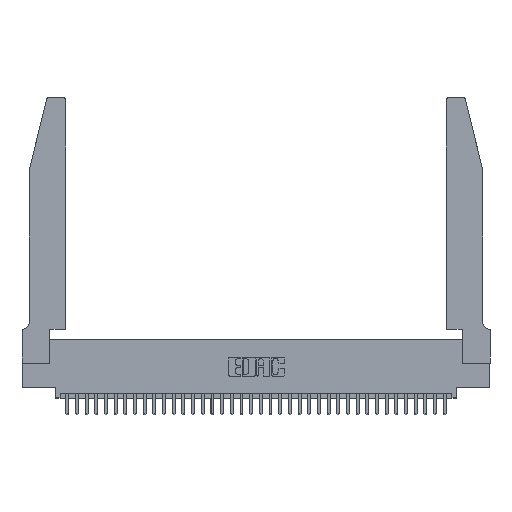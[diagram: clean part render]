
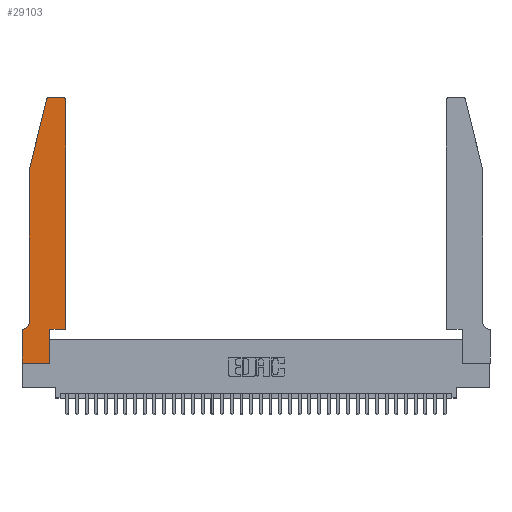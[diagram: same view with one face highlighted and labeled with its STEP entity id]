
A CAD part, top view. The second image highlights one B-rep face of the part: STEP entity #29103.
In plain terms, the highlighted planar face has unit normal (0, 0, 1).
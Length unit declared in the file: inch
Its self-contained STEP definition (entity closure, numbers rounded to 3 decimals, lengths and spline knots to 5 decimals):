
#94 = DIRECTION ( 'NONE',  ( -1., 0., 0. ) ) ;
#279 = CIRCLE ( 'NONE', #34975, 0.03 ) ;
#625 = FACE_OUTER_BOUND ( 'NONE', #15405, .T. ) ;
#995 = CARTESIAN_POINT ( 'NONE',  ( 0.0755, 2., 0.37 ) ) ;
#1442 = VECTOR ( 'NONE', #24357, 39.37008 ) ;
#2743 = DIRECTION ( 'NONE',  ( 0., 0., 1. ) ) ;
#3108 = CARTESIAN_POINT ( 'NONE',  ( 0.0755, 0.42, 0.37 ) ) ;
#3677 = LINE ( 'NONE', #20030, #7266 ) ;
#3759 = LINE ( 'NONE', #19079, #30808 ) ;
#3916 = LINE ( 'NONE', #7565, #27841 ) ;
#4178 = AXIS2_PLACEMENT_3D ( 'NONE', #19629, #25733, #22561 ) ;
#4283 = DIRECTION ( 'NONE',  ( 1., 0., 0. ) ) ;
#4795 = AXIS2_PLACEMENT_3D ( 'NONE', #17708, #6843, #6454 ) ;
#5957 = VECTOR ( 'NONE', #19794, 39.37008 ) ;
#6454 = DIRECTION ( 'NONE',  ( -1., 0., 0. ) ) ;
#6843 = DIRECTION ( 'NONE',  ( 0., 0., -1. ) ) ;
#7266 = VECTOR ( 'NONE', #11717, 39.37008 ) ;
#7565 = CARTESIAN_POINT ( 'NONE',  ( 0.4505, 0.35, 0.37 ) ) ;
#8391 = VERTEX_POINT ( 'NONE', #36003 ) ;
#9439 = EDGE_CURVE ( 'NONE', #10464, #17685, #34648, .T. ) ;
#9885 = DIRECTION ( 'NONE',  ( 0., 1., 0. ) ) ;
#10156 = ORIENTED_EDGE ( 'NONE', *, *, #19730, .T. ) ;
#10464 = VERTEX_POINT ( 'NONE', #36129 ) ;
#10573 = ORIENTED_EDGE ( 'NONE', *, *, #26274, .T. ) ;
#10985 = ORIENTED_EDGE ( 'NONE', *, *, #24171, .T. ) ;
#11085 = LINE ( 'NONE', #34331, #11903 ) ;
#11710 = ORIENTED_EDGE ( 'NONE', *, *, #30419, .T. ) ;
#11717 = DIRECTION ( 'NONE',  ( -1., 0., 0. ) ) ;
#11903 = VECTOR ( 'NONE', #17956, 39.37008 ) ;
#12091 = ORIENTED_EDGE ( 'NONE', *, *, #30946, .T. ) ;
#12439 = CARTESIAN_POINT ( 'NONE',  ( 0.4505, 0.35, 0.37 ) ) ;
#12511 = EDGE_CURVE ( 'NONE', #17685, #28322, #3916, .T. ) ;
#12722 = VERTEX_POINT ( 'NONE', #17600 ) ;
#12914 = LINE ( 'NONE', #30201, #31939 ) ;
#13151 = DIRECTION ( 'NONE',  ( 0., -1., 0. ) ) ;
#13572 = CARTESIAN_POINT ( 'NONE',  ( 0.25487, 2.72718, 0.37 ) ) ;
#13849 = DIRECTION ( 'NONE',  ( 1., 0., 0. ) ) ;
#13865 = CIRCLE ( 'NONE', #4795, 0.07 ) ;
#13953 = CARTESIAN_POINT ( 'NONE',  ( 0.284, 2.72, 0.37 ) ) ;
#14131 = VECTOR ( 'NONE', #94, 39.37008 ) ;
#14775 = EDGE_CURVE ( 'NONE', #35004, #17562, #3759, .T. ) ;
#15405 = EDGE_LOOP ( 'NONE', ( #11710, #12091, #22110, #30560, #10985, #10573, #32039, #10156, #29866, #31590, #23217, #34925 ) ) ;
#16206 = DIRECTION ( 'NONE',  ( -0.239, -0.971, 0. ) ) ;
#16333 = CARTESIAN_POINT ( 'NONE',  ( 0.0055, 0.35, 0.37 ) ) ;
#16591 = CARTESIAN_POINT ( 'NONE',  ( 0., 0.35, 0.37 ) ) ;
#16784 = VERTEX_POINT ( 'NONE', #16333 ) ;
#17246 = CARTESIAN_POINT ( 'NONE',  ( 0.0755, 0.35, 0.37 ) ) ;
#17562 = VERTEX_POINT ( 'NONE', #995 ) ;
#17600 = CARTESIAN_POINT ( 'NONE',  ( 0.4205, 2.75, 0.37 ) ) ;
#17685 = VERTEX_POINT ( 'NONE', #12439 ) ;
#17708 = CARTESIAN_POINT ( 'NONE',  ( 0.0055, 0.42, 0.37 ) ) ;
#17956 = DIRECTION ( 'NONE',  ( 0., 1., 0. ) ) ;
#18229 = EDGE_CURVE ( 'NONE', #28322, #12722, #279, .T. ) ;
#18492 = CARTESIAN_POINT ( 'NONE',  ( 0.4205, 2.72, 0.37 ) ) ;
#18801 = CARTESIAN_POINT ( 'NONE',  ( 0., 0., 0.37 ) ) ;
#19079 = CARTESIAN_POINT ( 'NONE',  ( 0.0755, 2., 0.37 ) ) ;
#19629 = CARTESIAN_POINT ( 'NONE',  ( 0., 0.35, 0.37 ) ) ;
#19730 = EDGE_CURVE ( 'NONE', #30642, #8391, #24966, .T. ) ;
#19794 = DIRECTION ( 'NONE',  ( 1., 0., 0. ) ) ;
#20030 = CARTESIAN_POINT ( 'NONE',  ( 0.2605, 2.75, 0.37 ) ) ;
#20596 = EDGE_CURVE ( 'NONE', #30633, #30642, #12914, .T. ) ;
#22110 = ORIENTED_EDGE ( 'NONE', *, *, #14775, .T. ) ;
#22561 = DIRECTION ( 'NONE',  ( 1., 0., 0. ) ) ;
#22845 = CARTESIAN_POINT ( 'NONE',  ( 0., 0., 0.37 ) ) ;
#23217 = ORIENTED_EDGE ( 'NONE', *, *, #12511, .T. ) ;
#24171 = EDGE_CURVE ( 'NONE', #34605, #16784, #13865, .T. ) ;
#24357 = DIRECTION ( 'NONE',  ( 1., 0., 0. ) ) ;
#24598 = AXIS2_PLACEMENT_3D ( 'NONE', #13953, #2743, #13849 ) ;
#24966 = LINE ( 'NONE', #22845, #5957 ) ;
#25733 = DIRECTION ( 'NONE',  ( 0., 0., 1. ) ) ;
#25803 = CIRCLE ( 'NONE', #24598, 0.03 ) ;
#25911 = LINE ( 'NONE', #29053, #26791 ) ;
#26274 = EDGE_CURVE ( 'NONE', #16784, #30633, #34487, .T. ) ;
#26468 = EDGE_CURVE ( 'NONE', #8391, #10464, #11085, .T. ) ;
#26791 = VECTOR ( 'NONE', #32005, 39.37008 ) ;
#27818 = CARTESIAN_POINT ( 'NONE',  ( 0.4505, 2.72, 0.37 ) ) ;
#27841 = VECTOR ( 'NONE', #9885, 39.37008 ) ;
#28138 = EDGE_CURVE ( 'NONE', #17562, #34605, #25911, .T. ) ;
#28322 = VERTEX_POINT ( 'NONE', #27818 ) ;
#28947 = CARTESIAN_POINT ( 'NONE',  ( 0.284, 2.75, 0.37 ) ) ;
#29053 = CARTESIAN_POINT ( 'NONE',  ( 0.0755, 2., 0.37 ) ) ;
#29103 = ADVANCED_FACE ( 'NONE', ( #625 ), #34204, .T. ) ;
#29866 = ORIENTED_EDGE ( 'NONE', *, *, #26468, .T. ) ;
#30201 = CARTESIAN_POINT ( 'NONE',  ( 0., 0., 0.37 ) ) ;
#30419 = EDGE_CURVE ( 'NONE', #12722, #35916, #3677, .T. ) ;
#30560 = ORIENTED_EDGE ( 'NONE', *, *, #28138, .T. ) ;
#30633 = VERTEX_POINT ( 'NONE', #16591 ) ;
#30642 = VERTEX_POINT ( 'NONE', #18801 ) ;
#30808 = VECTOR ( 'NONE', #16206, 39.37008 ) ;
#30946 = EDGE_CURVE ( 'NONE', #35916, #35004, #25803, .T. ) ;
#31590 = ORIENTED_EDGE ( 'NONE', *, *, #9439, .T. ) ;
#31939 = VECTOR ( 'NONE', #13151, 39.37008 ) ;
#32005 = DIRECTION ( 'NONE',  ( 0., -1., 0. ) ) ;
#32039 = ORIENTED_EDGE ( 'NONE', *, *, #20596, .T. ) ;
#32284 = CARTESIAN_POINT ( 'NONE',  ( 0.4505, 0.35, 0.37 ) ) ;
#32723 = DIRECTION ( 'NONE',  ( 0., 0., 1. ) ) ;
#34204 = PLANE ( 'NONE',  #4178 ) ;
#34331 = CARTESIAN_POINT ( 'NONE',  ( 0.2865, 0.35, 0.37 ) ) ;
#34487 = LINE ( 'NONE', #17246, #14131 ) ;
#34605 = VERTEX_POINT ( 'NONE', #3108 ) ;
#34648 = LINE ( 'NONE', #32284, #1442 ) ;
#34925 = ORIENTED_EDGE ( 'NONE', *, *, #18229, .T. ) ;
#34975 = AXIS2_PLACEMENT_3D ( 'NONE', #18492, #32723, #4283 ) ;
#35004 = VERTEX_POINT ( 'NONE', #13572 ) ;
#35916 = VERTEX_POINT ( 'NONE', #28947 ) ;
#36003 = CARTESIAN_POINT ( 'NONE',  ( 0.2865, 0., 0.37 ) ) ;
#36129 = CARTESIAN_POINT ( 'NONE',  ( 0.2865, 0.35, 0.37 ) ) ;
